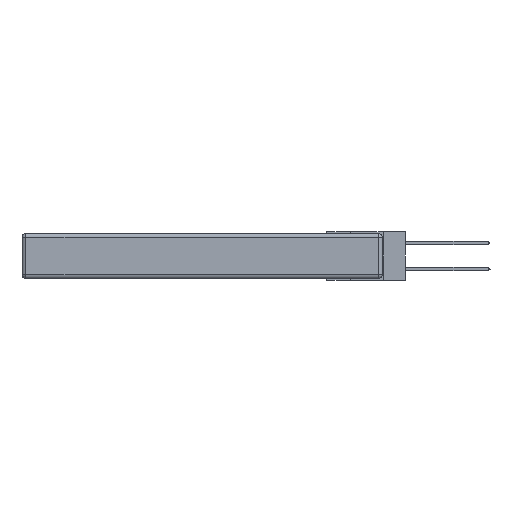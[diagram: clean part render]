
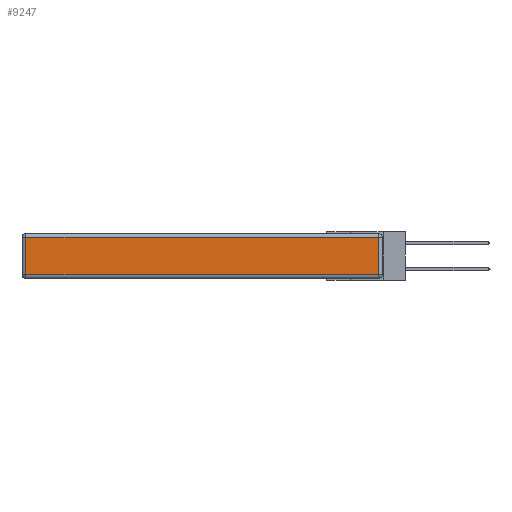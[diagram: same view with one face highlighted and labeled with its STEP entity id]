
A CAD part, left-side view. The second image highlights one B-rep face of the part: STEP entity #9247.
In plain terms, the highlighted planar face has unit normal (-1, 0, 0).
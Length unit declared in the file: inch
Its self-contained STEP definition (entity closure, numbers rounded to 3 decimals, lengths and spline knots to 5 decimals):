
#422 = ORIENTED_EDGE ( 'NONE', *, *, #5536, .T. ) ;
#1375 = VECTOR ( 'NONE', #9711, 39.37008 ) ;
#1534 = CARTESIAN_POINT ( 'NONE',  ( 0., 0., -0.313 ) ) ;
#1976 = DIRECTION ( 'NONE',  ( 0., 1., 0. ) ) ;
#2007 = DIRECTION ( 'NONE',  ( -1., 0., 0. ) ) ;
#2131 = DIRECTION ( 'NONE',  ( 0., 0., 1. ) ) ;
#2707 = LINE ( 'NONE', #5008, #4010 ) ;
#3577 = EDGE_LOOP ( 'NONE', ( #422, #6587, #3747, #9401 ) ) ;
#3747 = ORIENTED_EDGE ( 'NONE', *, *, #10840, .T. ) ;
#4010 = VECTOR ( 'NONE', #1976, 39.37008 ) ;
#4196 = CARTESIAN_POINT ( 'NONE',  ( 0., 0.03, -0.03 ) ) ;
#4907 = CARTESIAN_POINT ( 'NONE',  ( 0., 0.03, -0.313 ) ) ;
#5008 = CARTESIAN_POINT ( 'NONE',  ( 0., 2.75, -0.03 ) ) ;
#5156 = CARTESIAN_POINT ( 'NONE',  ( 0., 2.72, -0.343 ) ) ;
#5536 = EDGE_CURVE ( 'NONE', #6729, #7338, #11379, .T. ) ;
#6067 = CARTESIAN_POINT ( 'NONE',  ( 0., 0., -0.343 ) ) ;
#6419 = CARTESIAN_POINT ( 'NONE',  ( 0., 2.72, -0.03 ) ) ;
#6587 = ORIENTED_EDGE ( 'NONE', *, *, #8961, .T. ) ;
#6729 = VERTEX_POINT ( 'NONE', #9454 ) ;
#7338 = VERTEX_POINT ( 'NONE', #4907 ) ;
#8548 = VERTEX_POINT ( 'NONE', #4196 ) ;
#8961 = EDGE_CURVE ( 'NONE', #7338, #8548, #17795, .T. ) ;
#9084 = DIRECTION ( 'NONE',  ( 0., 0., 1. ) ) ;
#9247 = ADVANCED_FACE ( 'NONE', ( #12714 ), #10304, .T. ) ;
#9401 = ORIENTED_EDGE ( 'NONE', *, *, #14435, .T. ) ;
#9454 = CARTESIAN_POINT ( 'NONE',  ( 0., 2.72, -0.313 ) ) ;
#9711 = DIRECTION ( 'NONE',  ( 0., -1., 0. ) ) ;
#10120 = VECTOR ( 'NONE', #2131, 39.37008 ) ;
#10277 = VERTEX_POINT ( 'NONE', #6419 ) ;
#10304 = PLANE ( 'NONE',  #15067 ) ;
#10840 = EDGE_CURVE ( 'NONE', #8548, #10277, #2707, .T. ) ;
#11094 = VECTOR ( 'NONE', #13394, 39.37008 ) ;
#11379 = LINE ( 'NONE', #1534, #1375 ) ;
#12060 = CARTESIAN_POINT ( 'NONE',  ( 0., 0.03, -0.343 ) ) ;
#12714 = FACE_OUTER_BOUND ( 'NONE', #3577, .T. ) ;
#13394 = DIRECTION ( 'NONE',  ( 0., 0., -1. ) ) ;
#13697 = LINE ( 'NONE', #5156, #11094 ) ;
#14435 = EDGE_CURVE ( 'NONE', #10277, #6729, #13697, .T. ) ;
#15067 = AXIS2_PLACEMENT_3D ( 'NONE', #6067, #2007, #9084 ) ;
#17795 = LINE ( 'NONE', #12060, #10120 ) ;
